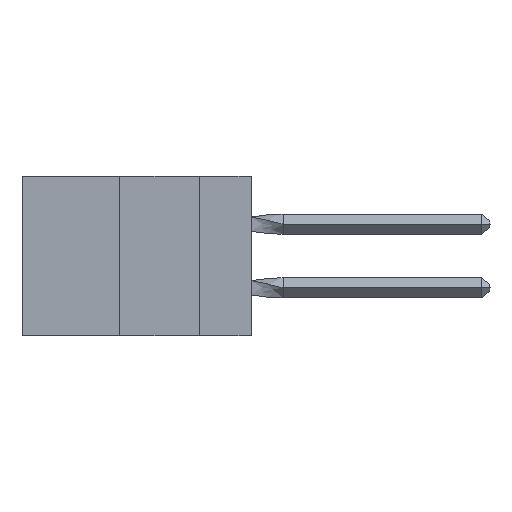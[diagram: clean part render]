
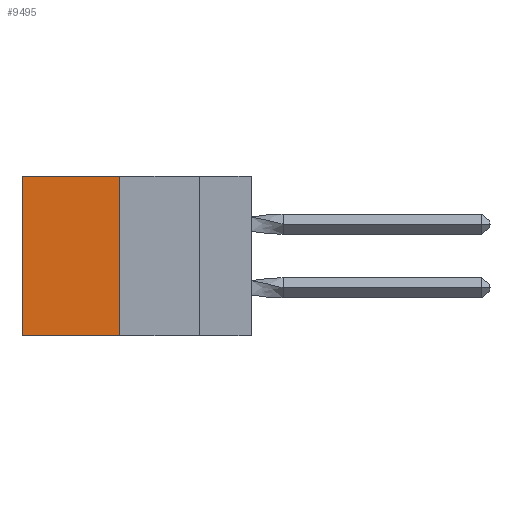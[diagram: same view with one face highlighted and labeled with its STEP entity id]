
A CAD part, left-side view. The second image highlights one B-rep face of the part: STEP entity #9495.
In plain terms, the highlighted planar face has unit normal (-1, 0, 0).
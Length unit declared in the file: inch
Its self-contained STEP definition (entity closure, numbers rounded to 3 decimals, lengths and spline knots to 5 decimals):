
#290 = VECTOR ( 'NONE', #22587, 39.37008 ) ;
#1469 = DIRECTION ( 'NONE',  ( 0., 1., 0. ) ) ;
#1894 = EDGE_CURVE ( 'NONE', #20460, #27940, #25343, .T. ) ;
#3979 = LINE ( 'NONE', #21053, #12730 ) ;
#4453 = EDGE_CURVE ( 'NONE', #27940, #10402, #3979, .T. ) ;
#4851 = CARTESIAN_POINT ( 'NONE',  ( 0.305, 0.72, -0.5 ) ) ;
#5002 = EDGE_CURVE ( 'NONE', #20460, #22658, #10399, .T. ) ;
#5066 = DIRECTION ( 'NONE',  ( 0., 0., -1. ) ) ;
#6305 = EDGE_LOOP ( 'NONE', ( #8822, #14357, #11468, #24426 ) ) ;
#6895 = CARTESIAN_POINT ( 'NONE',  ( 0.305, 0.413, -0.5 ) ) ;
#7746 = CARTESIAN_POINT ( 'NONE',  ( 0.305, 0.413, -0.5 ) ) ;
#8020 = PLANE ( 'NONE',  #9355 ) ;
#8822 = ORIENTED_EDGE ( 'NONE', *, *, #14420, .T. ) ;
#9355 = AXIS2_PLACEMENT_3D ( 'NONE', #16643, #25040, #27217 ) ;
#9495 = ADVANCED_FACE ( 'NONE', ( #23671 ), #8020, .F. ) ;
#9688 = CARTESIAN_POINT ( 'NONE',  ( 0.305, 0.413, 0. ) ) ;
#10399 = LINE ( 'NONE', #9688, #290 ) ;
#10402 = VERTEX_POINT ( 'NONE', #4851 ) ;
#11468 = ORIENTED_EDGE ( 'NONE', *, *, #1894, .F. ) ;
#12730 = VECTOR ( 'NONE', #1469, 39.37008 ) ;
#14281 = DIRECTION ( 'NONE',  ( 0., 0., -1. ) ) ;
#14357 = ORIENTED_EDGE ( 'NONE', *, *, #4453, .F. ) ;
#14420 = EDGE_CURVE ( 'NONE', #22658, #10402, #18115, .T. ) ;
#16643 = CARTESIAN_POINT ( 'NONE',  ( 0.305, 0.413, -0.5 ) ) ;
#18115 = LINE ( 'NONE', #22121, #27586 ) ;
#20460 = VERTEX_POINT ( 'NONE', #27209 ) ;
#20667 = CARTESIAN_POINT ( 'NONE',  ( 0.305, 0.72, 0. ) ) ;
#21053 = CARTESIAN_POINT ( 'NONE',  ( 0.305, 0.413, -0.5 ) ) ;
#22121 = CARTESIAN_POINT ( 'NONE',  ( 0.305, 0.72, -0.5 ) ) ;
#22587 = DIRECTION ( 'NONE',  ( 0., 1., 0. ) ) ;
#22649 = VECTOR ( 'NONE', #14281, 39.37008 ) ;
#22658 = VERTEX_POINT ( 'NONE', #20667 ) ;
#23671 = FACE_OUTER_BOUND ( 'NONE', #6305, .T. ) ;
#24426 = ORIENTED_EDGE ( 'NONE', *, *, #5002, .T. ) ;
#25040 = DIRECTION ( 'NONE',  ( 1., 0., 0. ) ) ;
#25343 = LINE ( 'NONE', #7746, #22649 ) ;
#27209 = CARTESIAN_POINT ( 'NONE',  ( 0.305, 0.413, 0. ) ) ;
#27217 = DIRECTION ( 'NONE',  ( 0., 0., -1. ) ) ;
#27586 = VECTOR ( 'NONE', #5066, 39.37008 ) ;
#27940 = VERTEX_POINT ( 'NONE', #6895 ) ;
